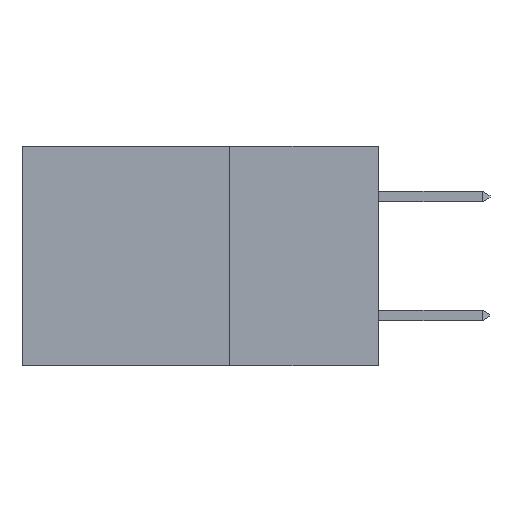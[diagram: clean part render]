
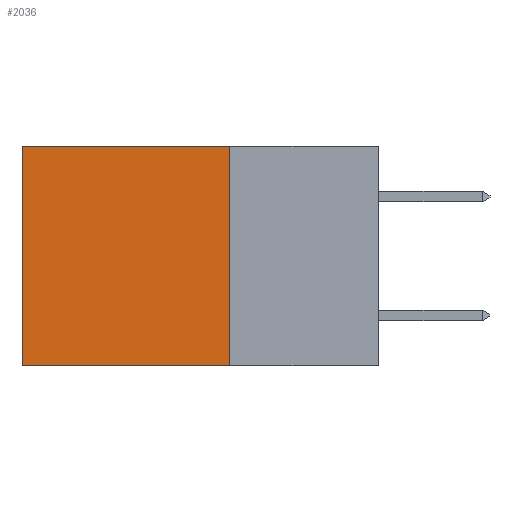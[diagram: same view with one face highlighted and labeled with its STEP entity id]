
A CAD part, left-side view. The second image highlights one B-rep face of the part: STEP entity #2036.
In plain terms, the highlighted planar face has unit normal (-1, 0, 0).
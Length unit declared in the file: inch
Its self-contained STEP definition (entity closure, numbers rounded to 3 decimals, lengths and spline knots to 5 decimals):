
#387 = ORIENTED_EDGE ( 'NONE', *, *, #4962, .F. ) ;
#529 = VERTEX_POINT ( 'NONE', #4284 ) ;
#2036 = ADVANCED_FACE ( 'NONE', ( #8737 ), #12635, .F. ) ;
#2436 = VERTEX_POINT ( 'NONE', #16351 ) ;
#2521 = VERTEX_POINT ( 'NONE', #9163 ) ;
#2641 = CARTESIAN_POINT ( 'NONE',  ( 0.298, 0.25, -0.37 ) ) ;
#4024 = DIRECTION ( 'NONE',  ( 0., 1., 0. ) ) ;
#4205 = ORIENTED_EDGE ( 'NONE', *, *, #14061, .F. ) ;
#4284 = CARTESIAN_POINT ( 'NONE',  ( 0.298, 0.6, -0.37 ) ) ;
#4539 = EDGE_CURVE ( 'NONE', #2436, #2521, #15977, .T. ) ;
#4962 = EDGE_CURVE ( 'NONE', #9433, #529, #6015, .T. ) ;
#4975 = DIRECTION ( 'NONE',  ( 0., 0., -1. ) ) ;
#5769 = LINE ( 'NONE', #14474, #8996 ) ;
#6015 = LINE ( 'NONE', #2641, #12877 ) ;
#7428 = ORIENTED_EDGE ( 'NONE', *, *, #15035, .T. ) ;
#8290 = AXIS2_PLACEMENT_3D ( 'NONE', #11328, #12615, #12612 ) ;
#8737 = FACE_OUTER_BOUND ( 'NONE', #14257, .T. ) ;
#8996 = VECTOR ( 'NONE', #4975, 39.37008 ) ;
#9163 = CARTESIAN_POINT ( 'NONE',  ( 0.298, 0.6, 0. ) ) ;
#9433 = VERTEX_POINT ( 'NONE', #9887 ) ;
#9887 = CARTESIAN_POINT ( 'NONE',  ( 0.298, 0.25, -0.37 ) ) ;
#10676 = DIRECTION ( 'NONE',  ( 0., 0., -1. ) ) ;
#11328 = CARTESIAN_POINT ( 'NONE',  ( 0.298, 0.25, 0. ) ) ;
#11464 = ORIENTED_EDGE ( 'NONE', *, *, #4539, .T. ) ;
#12456 = VECTOR ( 'NONE', #16496, 39.37008 ) ;
#12569 = VECTOR ( 'NONE', #10676, 39.37008 ) ;
#12612 = DIRECTION ( 'NONE',  ( 0., 0., -1. ) ) ;
#12615 = DIRECTION ( 'NONE',  ( 1., 0., 0. ) ) ;
#12635 = PLANE ( 'NONE',  #8290 ) ;
#12877 = VECTOR ( 'NONE', #4024, 39.37008 ) ;
#14061 = EDGE_CURVE ( 'NONE', #2436, #9433, #5769, .T. ) ;
#14257 = EDGE_LOOP ( 'NONE', ( #7428, #387, #4205, #11464 ) ) ;
#14474 = CARTESIAN_POINT ( 'NONE',  ( 0.298, 0.25, 0. ) ) ;
#15035 = EDGE_CURVE ( 'NONE', #2521, #529, #16091, .T. ) ;
#15192 = CARTESIAN_POINT ( 'NONE',  ( 0.298, 0.25, 0. ) ) ;
#15977 = LINE ( 'NONE', #15192, #12456 ) ;
#16091 = LINE ( 'NONE', #17295, #12569 ) ;
#16351 = CARTESIAN_POINT ( 'NONE',  ( 0.298, 0.25, 0. ) ) ;
#16496 = DIRECTION ( 'NONE',  ( 0., 1., 0. ) ) ;
#17295 = CARTESIAN_POINT ( 'NONE',  ( 0.298, 0.6, 0. ) ) ;
